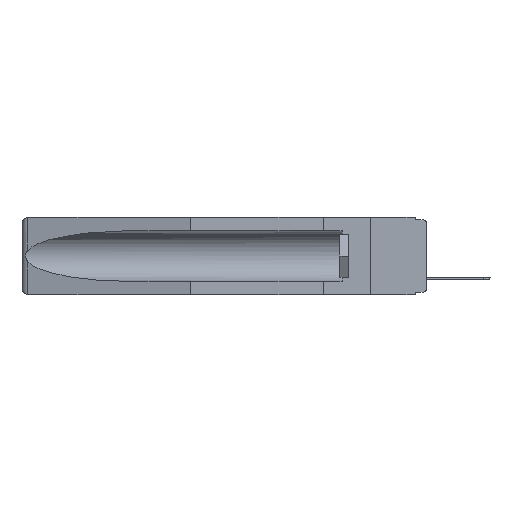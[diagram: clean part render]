
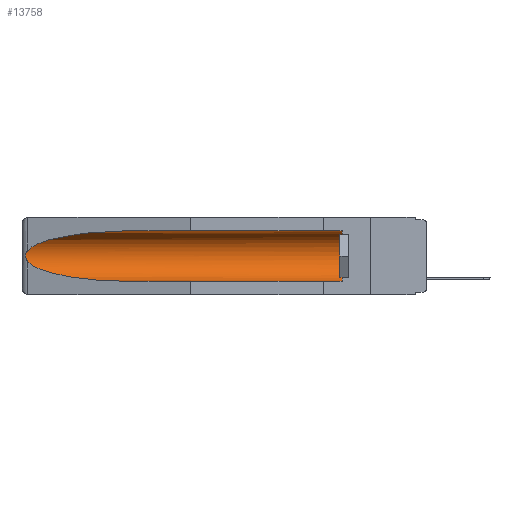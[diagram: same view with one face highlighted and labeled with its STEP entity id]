
A CAD part, left-side view. The second image highlights one B-rep face of the part: STEP entity #13758.
In plain terms, the highlighted cylindrical face has radius 2.857 mm (diameter 5.715 mm), a partial arc.
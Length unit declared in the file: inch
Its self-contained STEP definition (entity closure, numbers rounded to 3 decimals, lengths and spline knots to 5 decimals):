
#110 = B_SPLINE_CURVE_WITH_KNOTS ( 'NONE', 3,
 ( #12168, #20838, #26846, #27113, #1677, #16405, #16486, #3752, #20483, #5891 ),
 .UNSPECIFIED., .F., .F.,
 ( 4, 2, 2, 2, 4 ),
 ( 0., 0.00029, 0.00058, 0.00087, 0.00117 ),
 .UNSPECIFIED. ) ;
#184 = ORIENTED_EDGE ( 'NONE', *, *, #19585, .T. ) ;
#236 = EDGE_CURVE ( 'NONE', #708, #16485, #16584, .T. ) ;
#319 = VECTOR ( 'NONE', #19376, 39.37008 ) ;
#708 = VERTEX_POINT ( 'NONE', #9593 ) ;
#985 = CARTESIAN_POINT ( 'NONE',  ( 0.155, 1.07973, -0.059 ) ) ;
#1054 = VECTOR ( 'NONE', #23370, 39.37008 ) ;
#1677 = CARTESIAN_POINT ( 'NONE',  ( 0.2675, 1.53308, -0.16763 ) ) ;
#2473 = AXIS2_PLACEMENT_3D ( 'NONE', #4189, #25423, #4362 ) ;
#2707 = FACE_OUTER_BOUND ( 'NONE', #24542, .T. ) ;
#3483 = EDGE_CURVE ( 'NONE', #20344, #18986, #12060, .T. ) ;
#3752 = CARTESIAN_POINT ( 'NONE',  ( 0.26655, 1.53094, -0.18657 ) ) ;
#4108 = CARTESIAN_POINT ( 'NONE',  ( 0.155, 1.07973, -0.284 ) ) ;
#4189 = CARTESIAN_POINT ( 'NONE',  ( 0.155, -0.30754, -0.1715 ) ) ;
#4362 = DIRECTION ( 'NONE',  ( 0., 0., 1. ) ) ;
#4583 = CARTESIAN_POINT ( 'NONE',  ( 0.155, -0.30754, -0.284 ) ) ;
#5288 = EDGE_CURVE ( 'NONE', #11467, #20344, #8078, .T. ) ;
#5891 = CARTESIAN_POINT ( 'NONE',  ( 0.26537, 1.52718, -0.19328 ) ) ;
#6149 = CARTESIAN_POINT ( 'NONE',  ( 0.26537, 1.52718, -0.19328 ) ) ;
#6170 = EDGE_CURVE ( 'NONE', #708, #11467, #14606, .T. ) ;
#6513 = CARTESIAN_POINT ( 'NONE',  ( 0.155, -0.30754, -0.059 ) ) ;
#8078 = LINE ( 'NONE', #6513, #1054 ) ;
#9593 = CARTESIAN_POINT ( 'NONE',  ( 0.155, 0.126, -0.284 ) ) ;
#10793 = CARTESIAN_POINT ( 'NONE',  ( 0.21114, 1.30732, -0.059 ) ) ;
#11467 = VERTEX_POINT ( 'NONE', #12175 ) ;
#12060 =( BOUNDED_CURVE ( )  B_SPLINE_CURVE ( 3, ( #15375, #10793, #21480, #13166 ),
 .UNSPECIFIED., .F., .F. ) 
 B_SPLINE_CURVE_WITH_KNOTS ( ( 4, 4 ),
 ( 4.71239, 6.08839 ),
 .UNSPECIFIED. ) 
 CURVE ( )  GEOMETRIC_REPRESENTATION_ITEM ( )  RATIONAL_B_SPLINE_CURVE ( ( 1., 0.848, 0.848, 1. ) ) 
 REPRESENTATION_ITEM ( '' )  );
#12168 = CARTESIAN_POINT ( 'NONE',  ( 0.26537, 1.52718, -0.14972 ) ) ;
#12175 = CARTESIAN_POINT ( 'NONE',  ( 0.155, 0.126, -0.059 ) ) ;
#12381 = ORIENTED_EDGE ( 'NONE', *, *, #236, .F. ) ;
#13166 = CARTESIAN_POINT ( 'NONE',  ( 0.26537, 1.52718, -0.14972 ) ) ;
#13491 = AXIS2_PLACEMENT_3D ( 'NONE', #15212, #23807, #23618 ) ;
#13758 = ADVANCED_FACE ( 'NONE', ( #2707 ), #26178, .F. ) ;
#14596 = EDGE_CURVE ( 'NONE', #21640, #16485, #26406, .T. ) ;
#14606 = CIRCLE ( 'NONE', #13491, 0.1125 ) ;
#15212 = CARTESIAN_POINT ( 'NONE',  ( 0.155, 0.126, -0.1715 ) ) ;
#15375 = CARTESIAN_POINT ( 'NONE',  ( 0.155, 1.07973, -0.059 ) ) ;
#16405 = CARTESIAN_POINT ( 'NONE',  ( 0.2675, 1.53308, -0.17534 ) ) ;
#16485 = VERTEX_POINT ( 'NONE', #26866 ) ;
#16486 = CARTESIAN_POINT ( 'NONE',  ( 0.2673, 1.53269, -0.17917 ) ) ;
#16584 = LINE ( 'NONE', #4583, #319 ) ;
#18273 = CARTESIAN_POINT ( 'NONE',  ( 0.26537, 1.52718, -0.19328 ) ) ;
#18986 = VERTEX_POINT ( 'NONE', #26720 ) ;
#19376 = DIRECTION ( 'NONE',  ( 0., 1., 0. ) ) ;
#19585 = EDGE_CURVE ( 'NONE', #18986, #21640, #110, .T. ) ;
#19981 = ORIENTED_EDGE ( 'NONE', *, *, #6170, .T. ) ;
#20344 = VERTEX_POINT ( 'NONE', #985 ) ;
#20483 = CARTESIAN_POINT ( 'NONE',  ( 0.26597, 1.5296, -0.19026 ) ) ;
#20706 = ORIENTED_EDGE ( 'NONE', *, *, #14596, .T. ) ;
#20838 = CARTESIAN_POINT ( 'NONE',  ( 0.26597, 1.52961, -0.15275 ) ) ;
#21480 = CARTESIAN_POINT ( 'NONE',  ( 0.25451, 1.48313, -0.09465 ) ) ;
#21640 = VERTEX_POINT ( 'NONE', #18273 ) ;
#21955 = ORIENTED_EDGE ( 'NONE', *, *, #5288, .T. ) ;
#23370 = DIRECTION ( 'NONE',  ( 0., 1., 0. ) ) ;
#23618 = DIRECTION ( 'NONE',  ( 0., 0., 1. ) ) ;
#23807 = DIRECTION ( 'NONE',  ( 0., -1., 0. ) ) ;
#24542 = EDGE_LOOP ( 'NONE', ( #26294, #184, #20706, #12381, #19981, #21955 ) ) ;
#25420 = CARTESIAN_POINT ( 'NONE',  ( 0.25451, 1.48313, -0.24835 ) ) ;
#25423 = DIRECTION ( 'NONE',  ( 0., 1., 0. ) ) ;
#26178 = CYLINDRICAL_SURFACE ( 'NONE', #2473, 0.1125 ) ;
#26294 = ORIENTED_EDGE ( 'NONE', *, *, #3483, .T. ) ;
#26406 =( BOUNDED_CURVE ( )  B_SPLINE_CURVE ( 3, ( #6149, #25420, #27286, #4108 ),
 .UNSPECIFIED., .F., .F. ) 
 B_SPLINE_CURVE_WITH_KNOTS ( ( 4, 4 ),
 ( 0.1948, 1.5708 ),
 .UNSPECIFIED. ) 
 CURVE ( )  GEOMETRIC_REPRESENTATION_ITEM ( )  RATIONAL_B_SPLINE_CURVE ( ( 1., 0.848, 0.848, 1. ) ) 
 REPRESENTATION_ITEM ( '' )  );
#26720 = CARTESIAN_POINT ( 'NONE',  ( 0.26537, 1.52718, -0.14972 ) ) ;
#26846 = CARTESIAN_POINT ( 'NONE',  ( 0.26654, 1.53092, -0.15636 ) ) ;
#26866 = CARTESIAN_POINT ( 'NONE',  ( 0.155, 1.07973, -0.284 ) ) ;
#27113 = CARTESIAN_POINT ( 'NONE',  ( 0.2673, 1.5327, -0.16383 ) ) ;
#27286 = CARTESIAN_POINT ( 'NONE',  ( 0.21114, 1.30732, -0.284 ) ) ;
